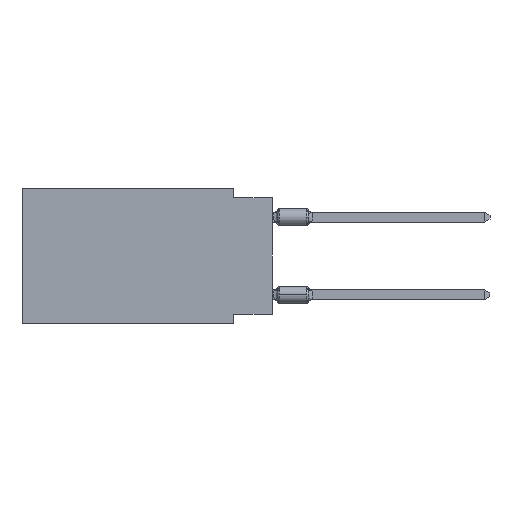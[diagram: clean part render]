
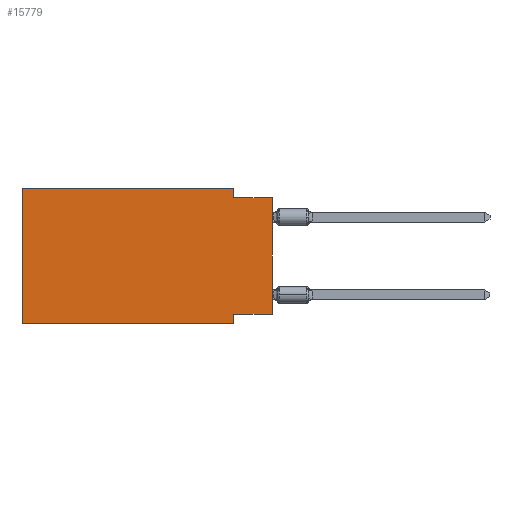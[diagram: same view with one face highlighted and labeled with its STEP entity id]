
A CAD part, left-side view. The second image highlights one B-rep face of the part: STEP entity #15779.
In plain terms, the highlighted planar face has unit normal (-1, 0, 0).
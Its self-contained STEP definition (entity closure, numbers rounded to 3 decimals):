
#281 = CARTESIAN_POINT ( 'NONE',  ( 0., 16.383, 0. ) ) ;
#504 = VECTOR ( 'NONE', #2969, 1000. ) ;
#1164 = CARTESIAN_POINT ( 'NONE',  ( 0., 16.383, 0. ) ) ;
#1502 = VECTOR ( 'NONE', #10847, 1000. ) ;
#1734 = LINE ( 'NONE', #14347, #19111 ) ;
#2415 = VECTOR ( 'NONE', #6915, 1000. ) ;
#2696 = VERTEX_POINT ( 'NONE', #15692 ) ;
#2701 = VECTOR ( 'NONE', #4583, 1000. ) ;
#2760 = DIRECTION ( 'NONE',  ( 0., 0., 1. ) ) ;
#2904 = CARTESIAN_POINT ( 'NONE',  ( 0., 2.54, -8.89 ) ) ;
#2969 = DIRECTION ( 'NONE',  ( 0., 0., -1. ) ) ;
#3341 = DIRECTION ( 'NONE',  ( 0., 0., -1. ) ) ;
#3464 = CARTESIAN_POINT ( 'NONE',  ( 0., 2.54, -8.89 ) ) ;
#4371 = ORIENTED_EDGE ( 'NONE', *, *, #10414, .F. ) ;
#4465 = FACE_OUTER_BOUND ( 'NONE', #6766, .T. ) ;
#4564 = LINE ( 'NONE', #9097, #11809 ) ;
#4583 = DIRECTION ( 'NONE',  ( 0., 1., 0. ) ) ;
#4858 = DIRECTION ( 'NONE',  ( 0., 0., 1. ) ) ;
#5059 = CARTESIAN_POINT ( 'NONE',  ( 0., 0., -0.635 ) ) ;
#5544 = EDGE_CURVE ( 'NONE', #17059, #15491, #14828, .T. ) ;
#5737 = EDGE_CURVE ( 'NONE', #10342, #12542, #9357, .T. ) ;
#5822 = CARTESIAN_POINT ( 'NONE',  ( 0., 0., -8.255 ) ) ;
#6431 = DIRECTION ( 'NONE',  ( 0., -1., 0. ) ) ;
#6605 = VERTEX_POINT ( 'NONE', #17860 ) ;
#6611 = ORIENTED_EDGE ( 'NONE', *, *, #5544, .T. ) ;
#6637 = AXIS2_PLACEMENT_3D ( 'NONE', #19597, #14961, #3341 ) ;
#6766 = EDGE_LOOP ( 'NONE', ( #18670, #7831, #11700, #13149, #15025, #6611, #8476, #4371 ) ) ;
#6915 = DIRECTION ( 'NONE',  ( 0., -1., 0. ) ) ;
#7491 = VECTOR ( 'NONE', #19675, 1000. ) ;
#7502 = LINE ( 'NONE', #12334, #504 ) ;
#7831 = ORIENTED_EDGE ( 'NONE', *, *, #15052, .F. ) ;
#8476 = ORIENTED_EDGE ( 'NONE', *, *, #16664, .F. ) ;
#8654 = VERTEX_POINT ( 'NONE', #5822 ) ;
#8798 = PLANE ( 'NONE',  #6637 ) ;
#9097 = CARTESIAN_POINT ( 'NONE',  ( 0., 16.383, 0. ) ) ;
#9229 = EDGE_CURVE ( 'NONE', #12542, #2696, #7502, .T. ) ;
#9357 = LINE ( 'NONE', #281, #18776 ) ;
#9490 = CARTESIAN_POINT ( 'NONE',  ( 0., 16.383, -8.89 ) ) ;
#10254 = LINE ( 'NONE', #2904, #1502 ) ;
#10342 = VERTEX_POINT ( 'NONE', #1164 ) ;
#10414 = EDGE_CURVE ( 'NONE', #8654, #6605, #12155, .T. ) ;
#10847 = DIRECTION ( 'NONE',  ( 0., 0., -1. ) ) ;
#11639 = CARTESIAN_POINT ( 'NONE',  ( 0., 0., -0.635 ) ) ;
#11700 = ORIENTED_EDGE ( 'NONE', *, *, #9229, .F. ) ;
#11809 = VECTOR ( 'NONE', #2760, 1000. ) ;
#12155 = LINE ( 'NONE', #16708, #2701 ) ;
#12334 = CARTESIAN_POINT ( 'NONE',  ( 0., 2.54, 0. ) ) ;
#12542 = VERTEX_POINT ( 'NONE', #16581 ) ;
#13149 = ORIENTED_EDGE ( 'NONE', *, *, #5737, .F. ) ;
#13308 = CARTESIAN_POINT ( 'NONE',  ( 0., 16.383, -8.89 ) ) ;
#14347 = CARTESIAN_POINT ( 'NONE',  ( 0., 0., 0. ) ) ;
#14783 = LINE ( 'NONE', #11639, #2415 ) ;
#14828 = LINE ( 'NONE', #13308, #7491 ) ;
#14961 = DIRECTION ( 'NONE',  ( 1., 0., 0. ) ) ;
#15025 = ORIENTED_EDGE ( 'NONE', *, *, #16954, .F. ) ;
#15052 = EDGE_CURVE ( 'NONE', #2696, #17154, #14783, .T. ) ;
#15491 = VERTEX_POINT ( 'NONE', #3464 ) ;
#15692 = CARTESIAN_POINT ( 'NONE',  ( 0., 2.54, -0.635 ) ) ;
#15779 = ADVANCED_FACE ( 'NONE', ( #4465 ), #8798, .F. ) ;
#16581 = CARTESIAN_POINT ( 'NONE',  ( 0., 2.54, 0. ) ) ;
#16664 = EDGE_CURVE ( 'NONE', #6605, #15491, #10254, .T. ) ;
#16708 = CARTESIAN_POINT ( 'NONE',  ( 0., 0., -8.255 ) ) ;
#16954 = EDGE_CURVE ( 'NONE', #17059, #10342, #4564, .T. ) ;
#17059 = VERTEX_POINT ( 'NONE', #9490 ) ;
#17154 = VERTEX_POINT ( 'NONE', #5059 ) ;
#17860 = CARTESIAN_POINT ( 'NONE',  ( 0., 2.54, -8.255 ) ) ;
#18670 = ORIENTED_EDGE ( 'NONE', *, *, #19809, .T. ) ;
#18776 = VECTOR ( 'NONE', #6431, 1000. ) ;
#19111 = VECTOR ( 'NONE', #4858, 1000. ) ;
#19597 = CARTESIAN_POINT ( 'NONE',  ( 0., 16.383, 0. ) ) ;
#19675 = DIRECTION ( 'NONE',  ( 0., -1., 0. ) ) ;
#19809 = EDGE_CURVE ( 'NONE', #8654, #17154, #1734, .T. ) ;
